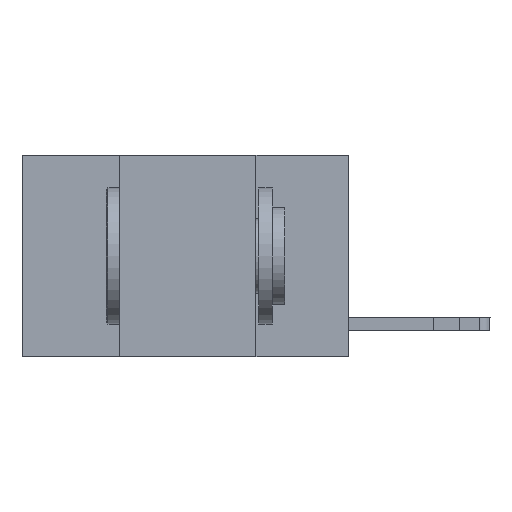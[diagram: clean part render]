
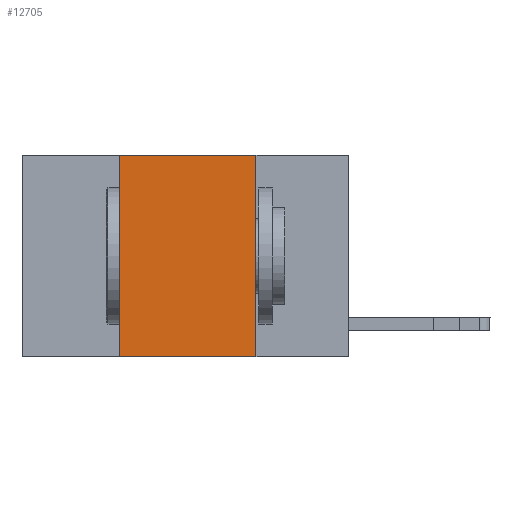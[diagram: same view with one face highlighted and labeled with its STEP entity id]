
A CAD part, left-side view. The second image highlights one B-rep face of the part: STEP entity #12705.
In plain terms, the highlighted planar face has unit normal (-1, 0, 0).
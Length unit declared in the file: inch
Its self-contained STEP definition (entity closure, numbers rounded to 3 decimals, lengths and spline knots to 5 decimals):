
#240 = VECTOR ( 'NONE', #18233, 39.37008 ) ;
#1932 = VECTOR ( 'NONE', #22641, 39.37008 ) ;
#2412 = DIRECTION ( 'NONE',  ( 0., 0., 1. ) ) ;
#2496 = VERTEX_POINT ( 'NONE', #6982 ) ;
#2851 = CARTESIAN_POINT ( 'NONE',  ( 0., 0.42, -0.37 ) ) ;
#3953 = CARTESIAN_POINT ( 'NONE',  ( 0., 0.17, 0. ) ) ;
#4038 = EDGE_CURVE ( 'NONE', #2496, #11110, #19807, .T. ) ;
#4944 = CARTESIAN_POINT ( 'NONE',  ( 0., 0.6, -0.37 ) ) ;
#5316 = VECTOR ( 'NONE', #2412, 39.37008 ) ;
#5883 = LINE ( 'NONE', #5962, #5316 ) ;
#5962 = CARTESIAN_POINT ( 'NONE',  ( 0., 0.42, 0. ) ) ;
#6655 = LINE ( 'NONE', #4944, #1932 ) ;
#6982 = CARTESIAN_POINT ( 'NONE',  ( 0., 0.17, 0. ) ) ;
#7359 = EDGE_LOOP ( 'NONE', ( #10090, #16425, #8415, #10665 ) ) ;
#7910 = PLANE ( 'NONE',  #15883 ) ;
#8415 = ORIENTED_EDGE ( 'NONE', *, *, #16555, .F. ) ;
#8501 = VECTOR ( 'NONE', #22024, 39.37008 ) ;
#8784 = EDGE_CURVE ( 'NONE', #11092, #11110, #6655, .T. ) ;
#9053 = LINE ( 'NONE', #16692, #8501 ) ;
#9926 = CARTESIAN_POINT ( 'NONE',  ( 0., 0.17, -0.37 ) ) ;
#10090 = ORIENTED_EDGE ( 'NONE', *, *, #4038, .F. ) ;
#10665 = ORIENTED_EDGE ( 'NONE', *, *, #8784, .T. ) ;
#11092 = VERTEX_POINT ( 'NONE', #2851 ) ;
#11110 = VERTEX_POINT ( 'NONE', #9926 ) ;
#11449 = DIRECTION ( 'NONE',  ( 0., 0., -1. ) ) ;
#12705 = ADVANCED_FACE ( 'NONE', ( #20952 ), #7910, .F. ) ;
#13879 = EDGE_CURVE ( 'NONE', #15908, #2496, #9053, .T. ) ;
#15883 = AXIS2_PLACEMENT_3D ( 'NONE', #20189, #21990, #11449 ) ;
#15908 = VERTEX_POINT ( 'NONE', #21960 ) ;
#16425 = ORIENTED_EDGE ( 'NONE', *, *, #13879, .F. ) ;
#16555 = EDGE_CURVE ( 'NONE', #11092, #15908, #5883, .T. ) ;
#16692 = CARTESIAN_POINT ( 'NONE',  ( 0., 0.6, 0. ) ) ;
#18233 = DIRECTION ( 'NONE',  ( 0., 0., -1. ) ) ;
#19807 = LINE ( 'NONE', #3953, #240 ) ;
#20189 = CARTESIAN_POINT ( 'NONE',  ( 0., 0.6, 0. ) ) ;
#20952 = FACE_OUTER_BOUND ( 'NONE', #7359, .T. ) ;
#21960 = CARTESIAN_POINT ( 'NONE',  ( 0., 0.42, 0. ) ) ;
#21990 = DIRECTION ( 'NONE',  ( 1., 0., 0. ) ) ;
#22024 = DIRECTION ( 'NONE',  ( 0., -1., 0. ) ) ;
#22641 = DIRECTION ( 'NONE',  ( 0., -1., 0. ) ) ;
